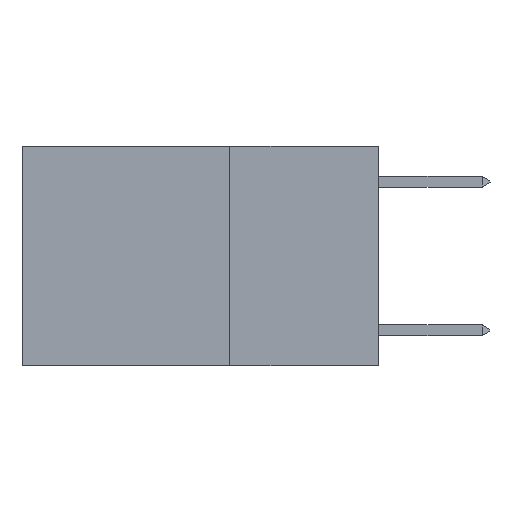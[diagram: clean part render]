
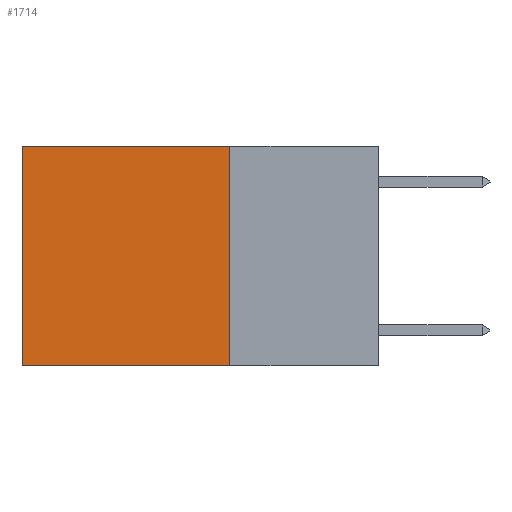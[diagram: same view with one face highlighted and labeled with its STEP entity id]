
A CAD part, left-side view. The second image highlights one B-rep face of the part: STEP entity #1714.
In plain terms, the highlighted planar face has unit normal (-1, 0, 0).
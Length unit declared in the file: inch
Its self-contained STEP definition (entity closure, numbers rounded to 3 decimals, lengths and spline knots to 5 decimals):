
#93 = DIRECTION ( 'NONE',  ( 0., 0., -1. ) ) ;
#94 = EDGE_CURVE ( 'NONE', #16279, #18722, #12698, .T. ) ;
#384 = VERTEX_POINT ( 'NONE', #20991 ) ;
#1538 = LINE ( 'NONE', #15372, #23960 ) ;
#1714 = ADVANCED_FACE ( 'NONE', ( #25975 ), #24618, .F. ) ;
#2369 = CARTESIAN_POINT ( 'NONE',  ( 0.2625, 0.25, 0. ) ) ;
#3446 = EDGE_LOOP ( 'NONE', ( #15681, #23685, #22853, #14303 ) ) ;
#3708 = CARTESIAN_POINT ( 'NONE',  ( 0.2625, 0.6, -0.37 ) ) ;
#3942 = DIRECTION ( 'NONE',  ( 0., 0., -1. ) ) ;
#4702 = LINE ( 'NONE', #8318, #7898 ) ;
#7432 = EDGE_CURVE ( 'NONE', #18722, #17694, #13589, .T. ) ;
#7854 = EDGE_CURVE ( 'NONE', #16279, #384, #4702, .T. ) ;
#7898 = VECTOR ( 'NONE', #3942, 39.37008 ) ;
#7926 = DIRECTION ( 'NONE',  ( 0., 0., -1. ) ) ;
#8199 = VECTOR ( 'NONE', #7926, 39.37008 ) ;
#8318 = CARTESIAN_POINT ( 'NONE',  ( 0.2625, 0.25, 0. ) ) ;
#11759 = DIRECTION ( 'NONE',  ( 0., 1., 0. ) ) ;
#12371 = DIRECTION ( 'NONE',  ( 1., 0., 0. ) ) ;
#12698 = LINE ( 'NONE', #16437, #21945 ) ;
#13589 = LINE ( 'NONE', #22371, #8199 ) ;
#13680 = AXIS2_PLACEMENT_3D ( 'NONE', #18355, #12371, #93 ) ;
#14303 = ORIENTED_EDGE ( 'NONE', *, *, #94, .T. ) ;
#15372 = CARTESIAN_POINT ( 'NONE',  ( 0.2625, 0.25, -0.37 ) ) ;
#15681 = ORIENTED_EDGE ( 'NONE', *, *, #7432, .T. ) ;
#16279 = VERTEX_POINT ( 'NONE', #2369 ) ;
#16437 = CARTESIAN_POINT ( 'NONE',  ( 0.2625, 0.25, 0. ) ) ;
#17694 = VERTEX_POINT ( 'NONE', #3708 ) ;
#18355 = CARTESIAN_POINT ( 'NONE',  ( 0.2625, 0.25, 0. ) ) ;
#18722 = VERTEX_POINT ( 'NONE', #25544 ) ;
#20991 = CARTESIAN_POINT ( 'NONE',  ( 0.2625, 0.25, -0.37 ) ) ;
#21945 = VECTOR ( 'NONE', #23101, 39.37008 ) ;
#22371 = CARTESIAN_POINT ( 'NONE',  ( 0.2625, 0.6, 0. ) ) ;
#22853 = ORIENTED_EDGE ( 'NONE', *, *, #7854, .F. ) ;
#23101 = DIRECTION ( 'NONE',  ( 0., 1., 0. ) ) ;
#23616 = EDGE_CURVE ( 'NONE', #384, #17694, #1538, .T. ) ;
#23685 = ORIENTED_EDGE ( 'NONE', *, *, #23616, .F. ) ;
#23960 = VECTOR ( 'NONE', #11759, 39.37008 ) ;
#24618 = PLANE ( 'NONE',  #13680 ) ;
#25544 = CARTESIAN_POINT ( 'NONE',  ( 0.2625, 0.6, 0. ) ) ;
#25975 = FACE_OUTER_BOUND ( 'NONE', #3446, .T. ) ;
